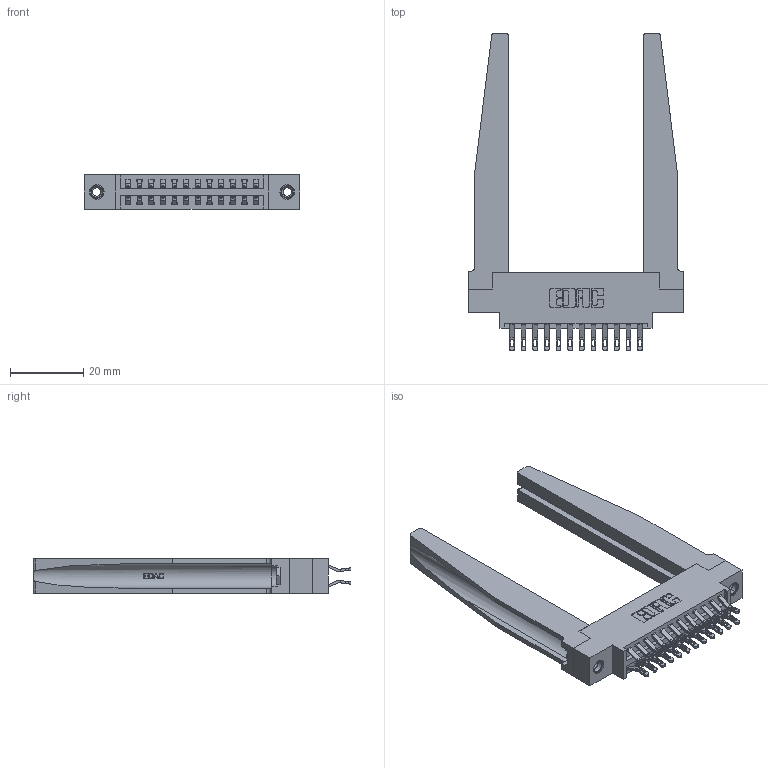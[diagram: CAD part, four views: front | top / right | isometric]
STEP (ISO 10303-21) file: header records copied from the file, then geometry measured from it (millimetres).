
FILE_DESCRIPTION (( 'STEP AP203' ), '1' );
FILE_NAME ('396-024-555-878.STEP', '2019-11-01T18:51:44', ( '' ), ( '' ), 'SwSTEP 2.0', 'SolidWorks 2016', '' );
FILE_SCHEMA (( 'CONFIG_CONTROL_DESIGN' ));
Length unit declared in the file: inch
Products named in the file (5): 346 Part_0.170 Offset - 0.156 Dia-TH; 345-292-001_555 Tail; 346-220-078_345-220-078; 345-250-001_345-250-001-102; 396-024-555-878
Assembly tree (29 placements, depth 2):
  396-024-555-878
    346 Part_0.170 Offset - 0.156 Dia-TH
    345-292-001_555 Tail  x24
    346-220-078_345-220-078  x2
    345-250-001_345-250-001-102  x2
Bounding box: 58.67 x 86.74 x 9.4 mm (x, y, z)
Volume: 12312.3 mm3; surface area: 13921.1 mm2
Topology: 29 solids, 29 shells, 1752 faces, 5341 edges, 3550 vertices
Faces by surface type: plane 1014, cylinder 686, bspline 36, cone 12, torus 4
Entity records: 17076 total; most frequent: CARTESIAN_POINT 3829, ORIENTED_EDGE 2622, DIRECTION 2381, EDGE_CURVE 1311, LINE 1017, VECTOR 1017, VERTEX_POINT 868, AXIS2_PLACEMENT_3D 682
